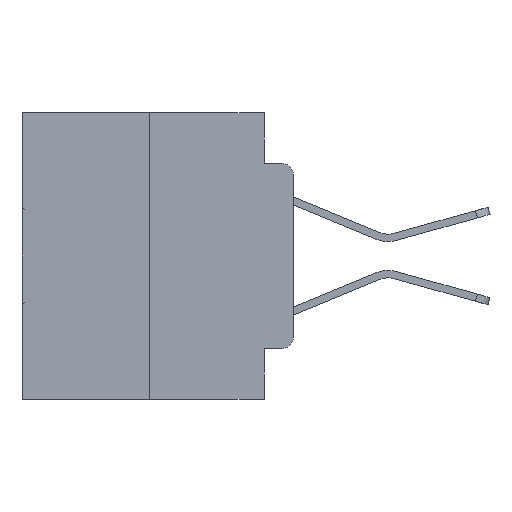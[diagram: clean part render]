
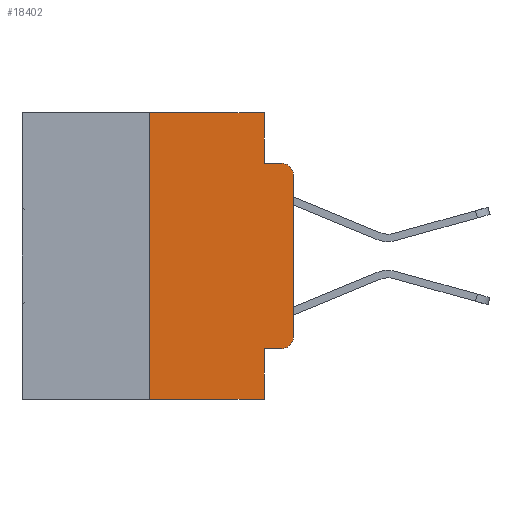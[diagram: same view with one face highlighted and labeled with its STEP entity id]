
A CAD part, left-side view. The second image highlights one B-rep face of the part: STEP entity #18402.
In plain terms, the highlighted planar face has unit normal (-1, 0, 0).
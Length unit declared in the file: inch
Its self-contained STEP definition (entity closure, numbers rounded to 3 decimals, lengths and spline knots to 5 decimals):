
#267 = ORIENTED_EDGE ( 'NONE', *, *, #26867, .T. ) ;
#647 = EDGE_CURVE ( 'NONE', #17128, #3509, #2070, .T. ) ;
#940 = CARTESIAN_POINT ( 'NONE',  ( 0., 0.051, -0.0885 ) ) ;
#1048 = DIRECTION ( 'NONE',  ( 0., 0., -1. ) ) ;
#2070 = LINE ( 'NONE', #18847, #24395 ) ;
#2169 = ORIENTED_EDGE ( 'NONE', *, *, #21390, .F. ) ;
#2240 = EDGE_CURVE ( 'NONE', #3509, #22697, #17927, .T. ) ;
#3509 = VERTEX_POINT ( 'NONE', #23687 ) ;
#3611 = CARTESIAN_POINT ( 'NONE',  ( 0., 0., 0. ) ) ;
#4341 = AXIS2_PLACEMENT_3D ( 'NONE', #6533, #22537, #8894 ) ;
#4843 = EDGE_CURVE ( 'NONE', #25048, #17974, #23001, .T. ) ;
#5491 = DIRECTION ( 'NONE',  ( 0., -1., 0. ) ) ;
#5981 = LINE ( 'NONE', #19381, #12154 ) ;
#6483 = DIRECTION ( 'NONE',  ( 0., -1., 0. ) ) ;
#6533 = CARTESIAN_POINT ( 'NONE',  ( 0., 0.02, -0.1085 ) ) ;
#6576 = ORIENTED_EDGE ( 'NONE', *, *, #2240, .F. ) ;
#7170 = CARTESIAN_POINT ( 'NONE',  ( 0., 0.25, 0. ) ) ;
#7342 = CARTESIAN_POINT ( 'NONE',  ( 0., 0.25, -0.5 ) ) ;
#7590 = EDGE_CURVE ( 'NONE', #11767, #25048, #26034, .T. ) ;
#7969 = CARTESIAN_POINT ( 'NONE',  ( 0., 0.051, -0.5 ) ) ;
#8894 = DIRECTION ( 'NONE',  ( 0., 0., -1. ) ) ;
#9137 = EDGE_CURVE ( 'NONE', #22630, #11767, #5981, .T. ) ;
#9161 = DIRECTION ( 'NONE',  ( -1., 0., 0. ) ) ;
#9183 = PLANE ( 'NONE',  #18677 ) ;
#10339 = CARTESIAN_POINT ( 'NONE',  ( 0., 0.25, 0. ) ) ;
#10932 = VECTOR ( 'NONE', #19011, 39.37008 ) ;
#11496 = DIRECTION ( 'NONE',  ( 0., 0., -1. ) ) ;
#11767 = VERTEX_POINT ( 'NONE', #16442 ) ;
#12154 = VECTOR ( 'NONE', #28347, 39.37008 ) ;
#14115 = EDGE_LOOP ( 'NONE', ( #29400, #267, #6576, #25518, #26935, #21635, #25897, #2169, #15251, #28723 ) ) ;
#14304 = VERTEX_POINT ( 'NONE', #10339 ) ;
#14919 = CARTESIAN_POINT ( 'NONE',  ( 0., 0.473, 0. ) ) ;
#15251 = ORIENTED_EDGE ( 'NONE', *, *, #9137, .T. ) ;
#15562 = CARTESIAN_POINT ( 'NONE',  ( 0., 0.051, 0. ) ) ;
#16237 = DIRECTION ( 'NONE',  ( 0., 0., 1. ) ) ;
#16297 = EDGE_CURVE ( 'NONE', #14304, #17128, #21401, .T. ) ;
#16401 = DIRECTION ( 'NONE',  ( 0., 0., -1. ) ) ;
#16408 = LINE ( 'NONE', #7170, #27728 ) ;
#16442 = CARTESIAN_POINT ( 'NONE',  ( 0., 0.02, -0.4115 ) ) ;
#17128 = VERTEX_POINT ( 'NONE', #15562 ) ;
#17927 = LINE ( 'NONE', #940, #23932 ) ;
#17974 = VERTEX_POINT ( 'NONE', #23637 ) ;
#18402 = ADVANCED_FACE ( 'NONE', ( #28669 ), #9183, .F. ) ;
#18677 = AXIS2_PLACEMENT_3D ( 'NONE', #22806, #25110, #11496 ) ;
#18847 = CARTESIAN_POINT ( 'NONE',  ( 0., 0.051, 0. ) ) ;
#19011 = DIRECTION ( 'NONE',  ( 0., 0., 1. ) ) ;
#19197 = LINE ( 'NONE', #20246, #25179 ) ;
#19381 = CARTESIAN_POINT ( 'NONE',  ( 0., 0.051, -0.4115 ) ) ;
#19709 = VECTOR ( 'NONE', #16401, 39.37008 ) ;
#20246 = CARTESIAN_POINT ( 'NONE',  ( 0., 0.473, -0.5 ) ) ;
#20314 = CARTESIAN_POINT ( 'NONE',  ( 0., 0.02, -0.0885 ) ) ;
#20413 = LINE ( 'NONE', #27667, #19709 ) ;
#21390 = EDGE_CURVE ( 'NONE', #22630, #23787, #20413, .T. ) ;
#21401 = LINE ( 'NONE', #14919, #26684 ) ;
#21635 = ORIENTED_EDGE ( 'NONE', *, *, #22862, .F. ) ;
#21763 = CARTESIAN_POINT ( 'NONE',  ( 0., 0., -0.3915 ) ) ;
#22537 = DIRECTION ( 'NONE',  ( -1., 0., 0. ) ) ;
#22630 = VERTEX_POINT ( 'NONE', #24463 ) ;
#22697 = VERTEX_POINT ( 'NONE', #20314 ) ;
#22785 = CARTESIAN_POINT ( 'NONE',  ( 0., 0.02, -0.3915 ) ) ;
#22806 = CARTESIAN_POINT ( 'NONE',  ( 0., 0.473, 0. ) ) ;
#22862 = EDGE_CURVE ( 'NONE', #23624, #14304, #16408, .T. ) ;
#23001 = LINE ( 'NONE', #3611, #10932 ) ;
#23624 = VERTEX_POINT ( 'NONE', #7342 ) ;
#23637 = CARTESIAN_POINT ( 'NONE',  ( 0., 0., -0.1085 ) ) ;
#23687 = CARTESIAN_POINT ( 'NONE',  ( 0., 0.051, -0.0885 ) ) ;
#23787 = VERTEX_POINT ( 'NONE', #7969 ) ;
#23932 = VECTOR ( 'NONE', #5491, 39.37008 ) ;
#24058 = EDGE_CURVE ( 'NONE', #23624, #23787, #19197, .T. ) ;
#24336 = CIRCLE ( 'NONE', #4341, 0.02 ) ;
#24395 = VECTOR ( 'NONE', #1048, 39.37008 ) ;
#24463 = CARTESIAN_POINT ( 'NONE',  ( 0., 0.051, -0.4115 ) ) ;
#24508 = AXIS2_PLACEMENT_3D ( 'NONE', #22785, #9161, #25088 ) ;
#25048 = VERTEX_POINT ( 'NONE', #21763 ) ;
#25088 = DIRECTION ( 'NONE',  ( 0., 0., -1. ) ) ;
#25110 = DIRECTION ( 'NONE',  ( 1., 0., 0. ) ) ;
#25179 = VECTOR ( 'NONE', #6483, 39.37008 ) ;
#25518 = ORIENTED_EDGE ( 'NONE', *, *, #647, .F. ) ;
#25897 = ORIENTED_EDGE ( 'NONE', *, *, #24058, .T. ) ;
#26034 = CIRCLE ( 'NONE', #24508, 0.02 ) ;
#26684 = VECTOR ( 'NONE', #28486, 39.37008 ) ;
#26867 = EDGE_CURVE ( 'NONE', #17974, #22697, #24336, .T. ) ;
#26935 = ORIENTED_EDGE ( 'NONE', *, *, #16297, .F. ) ;
#27667 = CARTESIAN_POINT ( 'NONE',  ( 0., 0.051, 0. ) ) ;
#27728 = VECTOR ( 'NONE', #16237, 39.37008 ) ;
#28347 = DIRECTION ( 'NONE',  ( 0., -1., 0. ) ) ;
#28486 = DIRECTION ( 'NONE',  ( 0., -1., 0. ) ) ;
#28669 = FACE_OUTER_BOUND ( 'NONE', #14115, .T. ) ;
#28723 = ORIENTED_EDGE ( 'NONE', *, *, #7590, .T. ) ;
#29400 = ORIENTED_EDGE ( 'NONE', *, *, #4843, .T. ) ;
